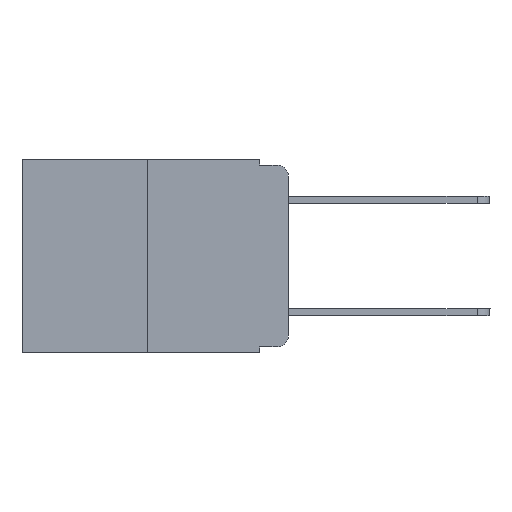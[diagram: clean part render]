
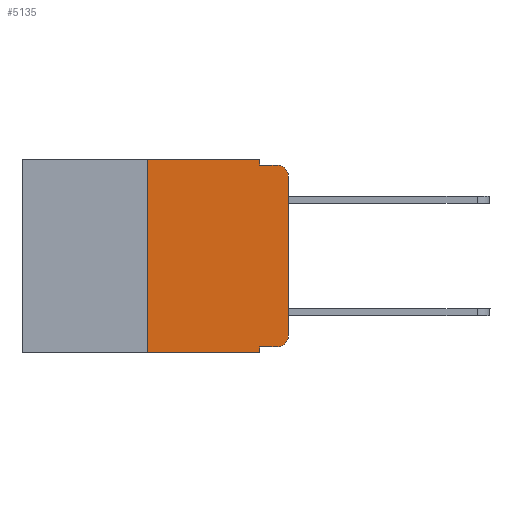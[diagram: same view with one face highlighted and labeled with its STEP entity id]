
A CAD part, left-side view. The second image highlights one B-rep face of the part: STEP entity #5135.
In plain terms, the highlighted planar face has unit normal (-1, 0, 0).
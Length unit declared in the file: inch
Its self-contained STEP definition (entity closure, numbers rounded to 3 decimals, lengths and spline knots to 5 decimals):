
#42 = VECTOR ( 'NONE', #4843, 39.37008 ) ;
#61 = DIRECTION ( 'NONE',  ( 0., 0., -1. ) ) ;
#190 = ORIENTED_EDGE ( 'NONE', *, *, #2000, .F. ) ;
#224 = CARTESIAN_POINT ( 'NONE',  ( 0., 0.25, 0. ) ) ;
#452 = CARTESIAN_POINT ( 'NONE',  ( 0., 0.051, -0.333 ) ) ;
#784 = LINE ( 'NONE', #224, #42 ) ;
#1300 = ORIENTED_EDGE ( 'NONE', *, *, #2813, .F. ) ;
#1341 = VERTEX_POINT ( 'NONE', #6160 ) ;
#1387 = CARTESIAN_POINT ( 'NONE',  ( 0., 0.02, -0.333 ) ) ;
#1501 = DIRECTION ( 'NONE',  ( 0., -1., 0. ) ) ;
#1989 = CARTESIAN_POINT ( 'NONE',  ( 0., 0.02, -0.03 ) ) ;
#2000 = EDGE_CURVE ( 'NONE', #3243, #4475, #8667, .T. ) ;
#2132 = DIRECTION ( 'NONE',  ( 0., 0., -1. ) ) ;
#2433 = VECTOR ( 'NONE', #6850, 39.37008 ) ;
#2813 = EDGE_CURVE ( 'NONE', #11107, #1341, #784, .T. ) ;
#2860 = DIRECTION ( 'NONE',  ( 0., 0., -1. ) ) ;
#3083 = LINE ( 'NONE', #5447, #9589 ) ;
#3243 = VERTEX_POINT ( 'NONE', #4709 ) ;
#3390 = EDGE_CURVE ( 'NONE', #12136, #9311, #9091, .T. ) ;
#3477 = VECTOR ( 'NONE', #4796, 39.37008 ) ;
#3863 = DIRECTION ( 'NONE',  ( 0., 0., 1. ) ) ;
#4004 = AXIS2_PLACEMENT_3D ( 'NONE', #1989, #8850, #61 ) ;
#4128 = VECTOR ( 'NONE', #2860, 39.37008 ) ;
#4301 = EDGE_CURVE ( 'NONE', #6014, #6652, #5265, .T. ) ;
#4469 = CARTESIAN_POINT ( 'NONE',  ( 0., 0., -0.313 ) ) ;
#4475 = VERTEX_POINT ( 'NONE', #9855 ) ;
#4546 = EDGE_CURVE ( 'NONE', #3243, #7815, #10701, .T. ) ;
#4709 = CARTESIAN_POINT ( 'NONE',  ( 0., 0.051, -0.333 ) ) ;
#4796 = DIRECTION ( 'NONE',  ( 0., -1., 0. ) ) ;
#4843 = DIRECTION ( 'NONE',  ( 0., 0., 1. ) ) ;
#5135 = ADVANCED_FACE ( 'NONE', ( #12174 ), #7920, .F. ) ;
#5175 = AXIS2_PLACEMENT_3D ( 'NONE', #9101, #8235, #11120 ) ;
#5265 = LINE ( 'NONE', #7749, #9823 ) ;
#5337 = CARTESIAN_POINT ( 'NONE',  ( 0., 0.02, -0.01 ) ) ;
#5447 = CARTESIAN_POINT ( 'NONE',  ( 0., 0.051, -0.01 ) ) ;
#5648 = EDGE_CURVE ( 'NONE', #6652, #8290, #10665, .T. ) ;
#6014 = VERTEX_POINT ( 'NONE', #4469 ) ;
#6160 = CARTESIAN_POINT ( 'NONE',  ( 0., 0.25, 0. ) ) ;
#6380 = ORIENTED_EDGE ( 'NONE', *, *, #7167, .F. ) ;
#6652 = VERTEX_POINT ( 'NONE', #7304 ) ;
#6693 = CARTESIAN_POINT ( 'NONE',  ( 0., 0.051, -0.01 ) ) ;
#6768 = CARTESIAN_POINT ( 'NONE',  ( 0., 0.473, 0. ) ) ;
#6850 = DIRECTION ( 'NONE',  ( 0., 0., -1. ) ) ;
#7070 = ORIENTED_EDGE ( 'NONE', *, *, #5648, .T. ) ;
#7167 = EDGE_CURVE ( 'NONE', #9311, #8290, #3083, .T. ) ;
#7304 = CARTESIAN_POINT ( 'NONE',  ( 0., 0., -0.03 ) ) ;
#7569 = CARTESIAN_POINT ( 'NONE',  ( 0., 0.473, -0.343 ) ) ;
#7658 = VECTOR ( 'NONE', #8546, 39.37008 ) ;
#7749 = CARTESIAN_POINT ( 'NONE',  ( 0., 0., 0. ) ) ;
#7761 = EDGE_CURVE ( 'NONE', #7815, #6014, #10710, .T. ) ;
#7812 = ORIENTED_EDGE ( 'NONE', *, *, #4301, .T. ) ;
#7815 = VERTEX_POINT ( 'NONE', #1387 ) ;
#7920 = PLANE ( 'NONE',  #9969 ) ;
#7967 = DIRECTION ( 'NONE',  ( 1., 0., 0. ) ) ;
#8081 = EDGE_CURVE ( 'NONE', #1341, #12136, #10850, .T. ) ;
#8235 = DIRECTION ( 'NONE',  ( -1., 0., 0. ) ) ;
#8290 = VERTEX_POINT ( 'NONE', #5337 ) ;
#8416 = LINE ( 'NONE', #7569, #7658 ) ;
#8546 = DIRECTION ( 'NONE',  ( 0., -1., 0. ) ) ;
#8667 = LINE ( 'NONE', #11491, #4128 ) ;
#8850 = DIRECTION ( 'NONE',  ( -1., 0., 0. ) ) ;
#8881 = CARTESIAN_POINT ( 'NONE',  ( 0., 0.051, 0. ) ) ;
#9034 = CARTESIAN_POINT ( 'NONE',  ( 0., 0.473, 0. ) ) ;
#9070 = VECTOR ( 'NONE', #9275, 39.37008 ) ;
#9091 = LINE ( 'NONE', #8881, #2433 ) ;
#9101 = CARTESIAN_POINT ( 'NONE',  ( 0., 0.02, -0.313 ) ) ;
#9117 = ORIENTED_EDGE ( 'NONE', *, *, #4546, .T. ) ;
#9275 = DIRECTION ( 'NONE',  ( 0., -1., 0. ) ) ;
#9311 = VERTEX_POINT ( 'NONE', #6693 ) ;
#9589 = VECTOR ( 'NONE', #1501, 39.37008 ) ;
#9783 = ORIENTED_EDGE ( 'NONE', *, *, #9939, .T. ) ;
#9823 = VECTOR ( 'NONE', #3863, 39.37008 ) ;
#9855 = CARTESIAN_POINT ( 'NONE',  ( 0., 0.051, -0.343 ) ) ;
#9939 = EDGE_CURVE ( 'NONE', #11107, #4475, #8416, .T. ) ;
#9969 = AXIS2_PLACEMENT_3D ( 'NONE', #9034, #7967, #2132 ) ;
#10457 = ORIENTED_EDGE ( 'NONE', *, *, #8081, .F. ) ;
#10665 = CIRCLE ( 'NONE', #4004, 0.02 ) ;
#10701 = LINE ( 'NONE', #452, #9070 ) ;
#10710 = CIRCLE ( 'NONE', #5175, 0.02 ) ;
#10850 = LINE ( 'NONE', #6768, #3477 ) ;
#10853 = CARTESIAN_POINT ( 'NONE',  ( 0., 0.25, -0.343 ) ) ;
#10959 = ORIENTED_EDGE ( 'NONE', *, *, #7761, .T. ) ;
#11107 = VERTEX_POINT ( 'NONE', #10853 ) ;
#11120 = DIRECTION ( 'NONE',  ( 0., 0., -1. ) ) ;
#11491 = CARTESIAN_POINT ( 'NONE',  ( 0., 0.051, 0. ) ) ;
#11541 = CARTESIAN_POINT ( 'NONE',  ( 0., 0.051, 0. ) ) ;
#11650 = ORIENTED_EDGE ( 'NONE', *, *, #3390, .F. ) ;
#12136 = VERTEX_POINT ( 'NONE', #11541 ) ;
#12170 = EDGE_LOOP ( 'NONE', ( #7812, #7070, #6380, #11650, #10457, #1300, #9783, #190, #9117, #10959 ) ) ;
#12174 = FACE_OUTER_BOUND ( 'NONE', #12170, .T. ) ;
